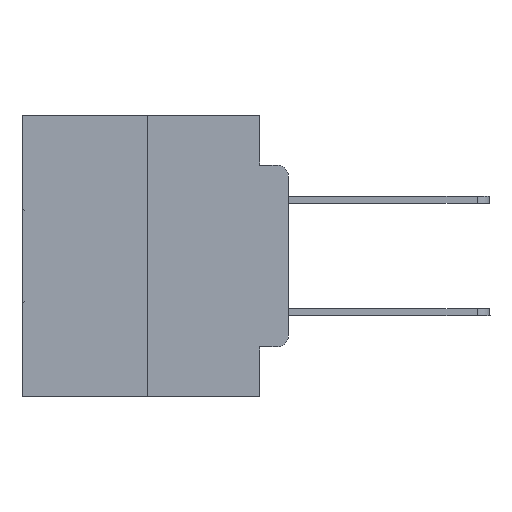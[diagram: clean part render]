
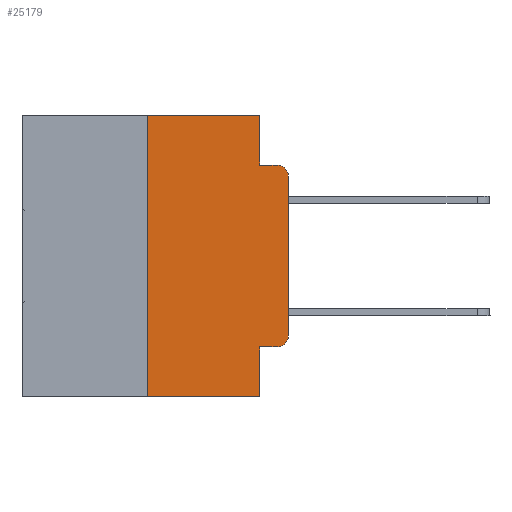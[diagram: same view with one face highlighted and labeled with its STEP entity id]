
A CAD part, left-side view. The second image highlights one B-rep face of the part: STEP entity #25179.
In plain terms, the highlighted planar face has unit normal (-1, 0, 0).
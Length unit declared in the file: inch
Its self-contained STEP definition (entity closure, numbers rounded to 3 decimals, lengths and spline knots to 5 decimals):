
#586 = EDGE_CURVE ( 'NONE', #2881, #17810, #2394, .T. ) ;
#1110 = EDGE_CURVE ( 'NONE', #31319, #2881, #20282, .T. ) ;
#1302 = LINE ( 'NONE', #9159, #23028 ) ;
#1551 = LINE ( 'NONE', #21330, #12965 ) ;
#2394 = LINE ( 'NONE', #11511, #19919 ) ;
#2421 = CIRCLE ( 'NONE', #3063, 0.02 ) ;
#2760 = EDGE_CURVE ( 'NONE', #28272, #7240, #15430, .T. ) ;
#2881 = VERTEX_POINT ( 'NONE', #18614 ) ;
#2900 = VECTOR ( 'NONE', #20434, 39.37008 ) ;
#3057 = CARTESIAN_POINT ( 'NONE',  ( 0., 0.051, 0. ) ) ;
#3063 = AXIS2_PLACEMENT_3D ( 'NONE', #22124, #7571, #24594 ) ;
#3694 = AXIS2_PLACEMENT_3D ( 'NONE', #9183, #4391, #21414 ) ;
#4096 = VECTOR ( 'NONE', #25743, 39.37008 ) ;
#4391 = DIRECTION ( 'NONE',  ( -1., 0., 0. ) ) ;
#4804 = CARTESIAN_POINT ( 'NONE',  ( 0., 0.473, 0. ) ) ;
#5479 = VERTEX_POINT ( 'NONE', #3057 ) ;
#5772 = EDGE_CURVE ( 'NONE', #23524, #31319, #1551, .T. ) ;
#5869 = EDGE_CURVE ( 'NONE', #23524, #15732, #17560, .T. ) ;
#7037 = LINE ( 'NONE', #7814, #12699 ) ;
#7240 = VERTEX_POINT ( 'NONE', #9621 ) ;
#7258 = PLANE ( 'NONE',  #10482 ) ;
#7325 = ORIENTED_EDGE ( 'NONE', *, *, #2760, .F. ) ;
#7375 = LINE ( 'NONE', #25738, #11165 ) ;
#7571 = DIRECTION ( 'NONE',  ( -1., 0., 0. ) ) ;
#7814 = CARTESIAN_POINT ( 'NONE',  ( 0., 0.25, 0. ) ) ;
#7851 = DIRECTION ( 'NONE',  ( 0., 0., -1. ) ) ;
#8499 = CARTESIAN_POINT ( 'NONE',  ( 0., 0.051, -0.5 ) ) ;
#8664 = ORIENTED_EDGE ( 'NONE', *, *, #5772, .T. ) ;
#8779 = EDGE_CURVE ( 'NONE', #9538, #15732, #1302, .T. ) ;
#9159 = CARTESIAN_POINT ( 'NONE',  ( 0., 0.473, -0.5 ) ) ;
#9173 = DIRECTION ( 'NONE',  ( 0., 0., 1. ) ) ;
#9183 = CARTESIAN_POINT ( 'NONE',  ( 0., 0.02, -0.3915 ) ) ;
#9210 = DIRECTION ( 'NONE',  ( 0., -1., 0. ) ) ;
#9274 = CARTESIAN_POINT ( 'NONE',  ( 0., 0.25, -0.5 ) ) ;
#9481 = EDGE_CURVE ( 'NONE', #17810, #7240, #2421, .T. ) ;
#9538 = VERTEX_POINT ( 'NONE', #9274 ) ;
#9621 = CARTESIAN_POINT ( 'NONE',  ( 0., 0.02, -0.0885 ) ) ;
#9703 = DIRECTION ( 'NONE',  ( 1., 0., 0. ) ) ;
#9889 = CARTESIAN_POINT ( 'NONE',  ( 0., 0.051, -0.4115 ) ) ;
#10448 = DIRECTION ( 'NONE',  ( 0., 0., 1. ) ) ;
#10482 = AXIS2_PLACEMENT_3D ( 'NONE', #4804, #9703, #7851 ) ;
#10827 = EDGE_LOOP ( 'NONE', ( #15953, #28442, #7325, #13276, #20747, #23835, #22069, #25289, #8664, #28230 ) ) ;
#11165 = VECTOR ( 'NONE', #15836, 39.37008 ) ;
#11511 = CARTESIAN_POINT ( 'NONE',  ( 0., 0., 0. ) ) ;
#12699 = VECTOR ( 'NONE', #10448, 39.37008 ) ;
#12965 = VECTOR ( 'NONE', #9210, 39.37008 ) ;
#13276 = ORIENTED_EDGE ( 'NONE', *, *, #21376, .F. ) ;
#14541 = VERTEX_POINT ( 'NONE', #20819 ) ;
#15430 = LINE ( 'NONE', #17784, #2900 ) ;
#15462 = CARTESIAN_POINT ( 'NONE',  ( 0., 0.02, -0.4115 ) ) ;
#15603 = EDGE_CURVE ( 'NONE', #9538, #14541, #7037, .T. ) ;
#15732 = VERTEX_POINT ( 'NONE', #8499 ) ;
#15836 = DIRECTION ( 'NONE',  ( 0., -1., 0. ) ) ;
#15953 = ORIENTED_EDGE ( 'NONE', *, *, #586, .T. ) ;
#17560 = LINE ( 'NONE', #31409, #25172 ) ;
#17784 = CARTESIAN_POINT ( 'NONE',  ( 0., 0.051, -0.0885 ) ) ;
#17810 = VERTEX_POINT ( 'NONE', #28767 ) ;
#18556 = LINE ( 'NONE', #28094, #4096 ) ;
#18614 = CARTESIAN_POINT ( 'NONE',  ( 0., 0., -0.3915 ) ) ;
#19919 = VECTOR ( 'NONE', #9173, 39.37008 ) ;
#20282 = CIRCLE ( 'NONE', #3694, 0.02 ) ;
#20434 = DIRECTION ( 'NONE',  ( 0., -1., 0. ) ) ;
#20747 = ORIENTED_EDGE ( 'NONE', *, *, #28671, .F. ) ;
#20819 = CARTESIAN_POINT ( 'NONE',  ( 0., 0.25, 0. ) ) ;
#21330 = CARTESIAN_POINT ( 'NONE',  ( 0., 0.051, -0.4115 ) ) ;
#21376 = EDGE_CURVE ( 'NONE', #5479, #28272, #18556, .T. ) ;
#21414 = DIRECTION ( 'NONE',  ( 0., 0., -1. ) ) ;
#21551 = DIRECTION ( 'NONE',  ( 0., 0., -1. ) ) ;
#22069 = ORIENTED_EDGE ( 'NONE', *, *, #8779, .T. ) ;
#22124 = CARTESIAN_POINT ( 'NONE',  ( 0., 0.02, -0.1085 ) ) ;
#23028 = VECTOR ( 'NONE', #26195, 39.37008 ) ;
#23524 = VERTEX_POINT ( 'NONE', #9889 ) ;
#23835 = ORIENTED_EDGE ( 'NONE', *, *, #15603, .F. ) ;
#24594 = DIRECTION ( 'NONE',  ( 0., 0., -1. ) ) ;
#25172 = VECTOR ( 'NONE', #21551, 39.37008 ) ;
#25179 = ADVANCED_FACE ( 'NONE', ( #29051 ), #7258, .F. ) ;
#25289 = ORIENTED_EDGE ( 'NONE', *, *, #5869, .F. ) ;
#25738 = CARTESIAN_POINT ( 'NONE',  ( 0., 0.473, 0. ) ) ;
#25743 = DIRECTION ( 'NONE',  ( 0., 0., -1. ) ) ;
#26195 = DIRECTION ( 'NONE',  ( 0., -1., 0. ) ) ;
#26523 = CARTESIAN_POINT ( 'NONE',  ( 0., 0.051, -0.0885 ) ) ;
#28094 = CARTESIAN_POINT ( 'NONE',  ( 0., 0.051, 0. ) ) ;
#28230 = ORIENTED_EDGE ( 'NONE', *, *, #1110, .T. ) ;
#28272 = VERTEX_POINT ( 'NONE', #26523 ) ;
#28442 = ORIENTED_EDGE ( 'NONE', *, *, #9481, .T. ) ;
#28671 = EDGE_CURVE ( 'NONE', #14541, #5479, #7375, .T. ) ;
#28767 = CARTESIAN_POINT ( 'NONE',  ( 0., 0., -0.1085 ) ) ;
#29051 = FACE_OUTER_BOUND ( 'NONE', #10827, .T. ) ;
#31319 = VERTEX_POINT ( 'NONE', #15462 ) ;
#31409 = CARTESIAN_POINT ( 'NONE',  ( 0., 0.051, 0. ) ) ;
